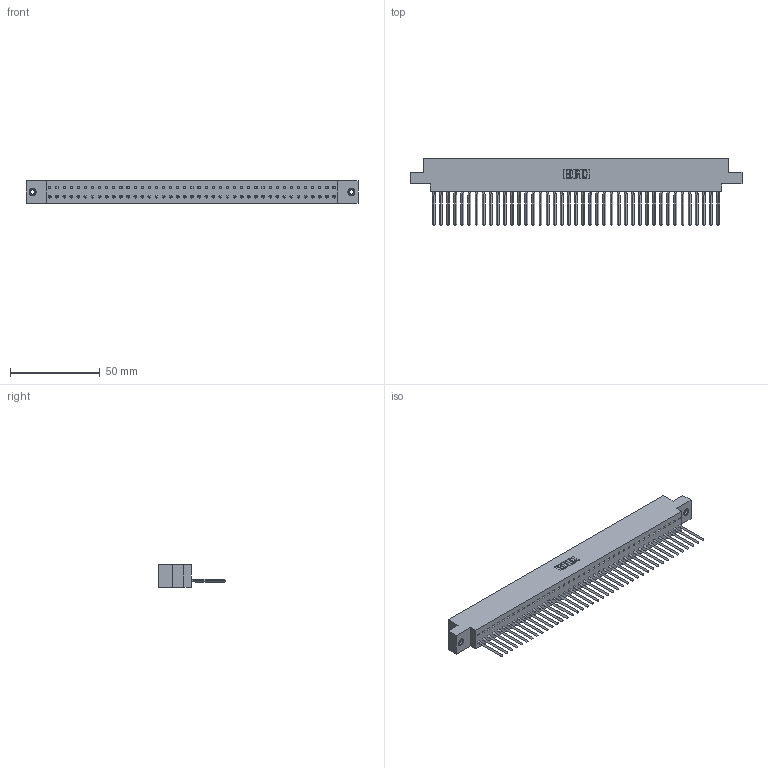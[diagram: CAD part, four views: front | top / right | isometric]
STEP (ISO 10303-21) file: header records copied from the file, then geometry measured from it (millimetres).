
FILE_DESCRIPTION (( 'STEP AP203' ), '1' );
FILE_NAME ('317-041-541-607.STEP', '2020-02-28T00:58:43', ( '' ), ( '' ), 'SwSTEP 2.0', 'SolidWorks 2016', '' );
FILE_SCHEMA (( 'CONFIG_CONTROL_DESIGN' ));
Length unit declared in the file: inch
Products named in the file (4): 317 Part_.156 Dia - TI; 345-250-001_345-250-005-103; 317-041-541-607; 317-290-002_541
Assembly tree (44 placements, depth 2):
  317-041-541-607
    317 Part_.156 Dia - TI
    317-290-002_541  x41
    345-250-001_345-250-005-103  x2
Bounding box: 185.17 x 37.34 x 12.7 mm (x, y, z)
Volume: 29983.4 mm3; surface area: 42370.8 mm2
Topology: 44 solids, 44 shells, 6394 faces, 18205 edges, 11828 vertices
Faces by surface type: plane 5174, cylinder 1040, bspline 164, cone 12, torus 4
Entity records: 60827 total; most frequent: CARTESIAN_POINT 11423, ORIENTED_EDGE 10710, DIRECTION 8839, EDGE_CURVE 5355, LINE 4971, VECTOR 4971, VERTEX_POINT 3558, AXIS2_PLACEMENT_3D 1934
